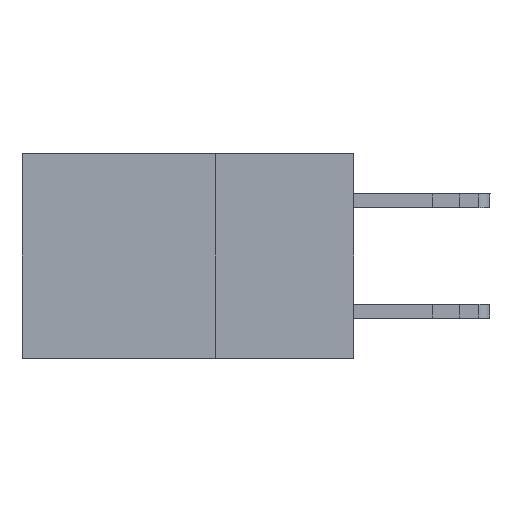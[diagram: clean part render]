
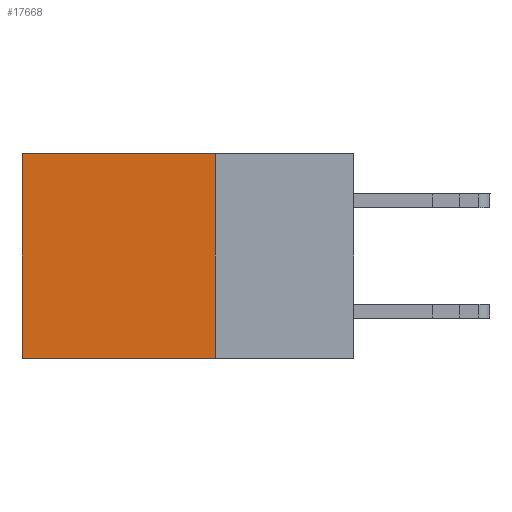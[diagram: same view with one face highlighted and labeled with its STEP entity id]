
A CAD part, left-side view. The second image highlights one B-rep face of the part: STEP entity #17668.
In plain terms, the highlighted planar face has unit normal (-1, 0, 0).
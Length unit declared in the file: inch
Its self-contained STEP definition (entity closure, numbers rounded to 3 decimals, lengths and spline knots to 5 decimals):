
#67 = LINE ( 'NONE', #26852, #10714 ) ;
#176 = DIRECTION ( 'NONE',  ( 0., 1., 0. ) ) ;
#1250 = DIRECTION ( 'NONE',  ( 1., 0., 0. ) ) ;
#1555 = CARTESIAN_POINT ( 'NONE',  ( 0.2875, 0.25, 0. ) ) ;
#1556 = PLANE ( 'NONE',  #25314 ) ;
#3005 = CARTESIAN_POINT ( 'NONE',  ( 0.2875, 0.25, 0. ) ) ;
#3800 = CARTESIAN_POINT ( 'NONE',  ( 0.2875, 0.25, 0. ) ) ;
#3840 = LINE ( 'NONE', #17520, #17562 ) ;
#4090 = CARTESIAN_POINT ( 'NONE',  ( 0.2875, 0.6, -0.37 ) ) ;
#4217 = VECTOR ( 'NONE', #10341, 39.37008 ) ;
#5465 = DIRECTION ( 'NONE',  ( 0., 0., -1. ) ) ;
#5748 = EDGE_LOOP ( 'NONE', ( #31276, #14657, #28235, #20863 ) ) ;
#8596 = DIRECTION ( 'NONE',  ( 0., 0., -1. ) ) ;
#9640 = EDGE_CURVE ( 'NONE', #15761, #29517, #17828, .T. ) ;
#10341 = DIRECTION ( 'NONE',  ( 0., 1., 0. ) ) ;
#10714 = VECTOR ( 'NONE', #176, 39.37008 ) ;
#12895 = CARTESIAN_POINT ( 'NONE',  ( 0.2875, 0.6, 0. ) ) ;
#14438 = EDGE_CURVE ( 'NONE', #23278, #29517, #67, .T. ) ;
#14657 = ORIENTED_EDGE ( 'NONE', *, *, #14438, .F. ) ;
#15761 = VERTEX_POINT ( 'NONE', #27216 ) ;
#17520 = CARTESIAN_POINT ( 'NONE',  ( 0.2875, 0.25, 0. ) ) ;
#17562 = VECTOR ( 'NONE', #22072, 39.37008 ) ;
#17668 = ADVANCED_FACE ( 'NONE', ( #20869 ), #1556, .F. ) ;
#17828 = LINE ( 'NONE', #12895, #19348 ) ;
#19348 = VECTOR ( 'NONE', #5465, 39.37008 ) ;
#20863 = ORIENTED_EDGE ( 'NONE', *, *, #28661, .T. ) ;
#20869 = FACE_OUTER_BOUND ( 'NONE', #5748, .T. ) ;
#21526 = EDGE_CURVE ( 'NONE', #23364, #23278, #3840, .T. ) ;
#21699 = LINE ( 'NONE', #3005, #4217 ) ;
#22072 = DIRECTION ( 'NONE',  ( 0., 0., -1. ) ) ;
#23278 = VERTEX_POINT ( 'NONE', #28247 ) ;
#23364 = VERTEX_POINT ( 'NONE', #1555 ) ;
#25314 = AXIS2_PLACEMENT_3D ( 'NONE', #3800, #1250, #8596 ) ;
#26852 = CARTESIAN_POINT ( 'NONE',  ( 0.2875, 0.25, -0.37 ) ) ;
#27216 = CARTESIAN_POINT ( 'NONE',  ( 0.2875, 0.6, 0. ) ) ;
#28235 = ORIENTED_EDGE ( 'NONE', *, *, #21526, .F. ) ;
#28247 = CARTESIAN_POINT ( 'NONE',  ( 0.2875, 0.25, -0.37 ) ) ;
#28661 = EDGE_CURVE ( 'NONE', #23364, #15761, #21699, .T. ) ;
#29517 = VERTEX_POINT ( 'NONE', #4090 ) ;
#31276 = ORIENTED_EDGE ( 'NONE', *, *, #9640, .T. ) ;
